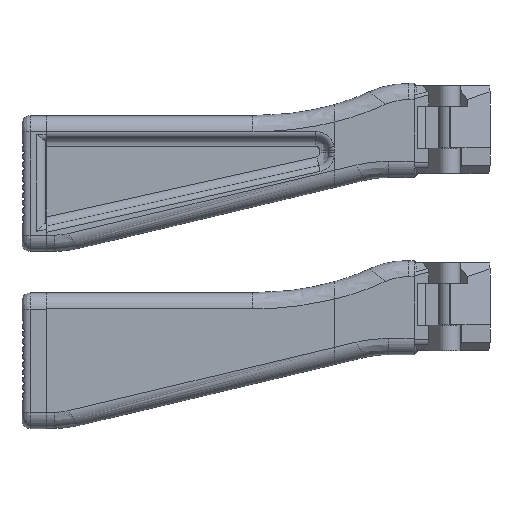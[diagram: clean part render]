
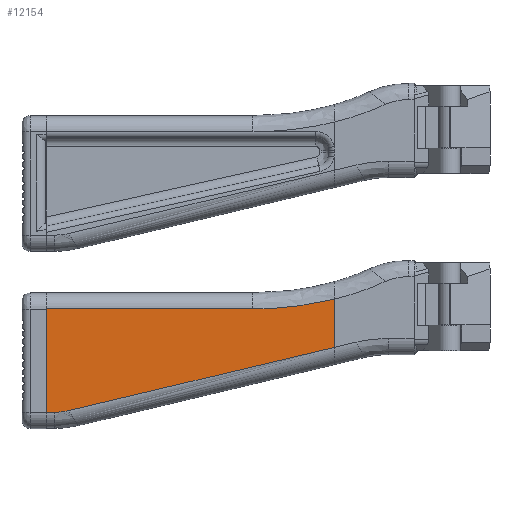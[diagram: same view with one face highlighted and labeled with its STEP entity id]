
A CAD part, top view. The second image highlights one B-rep face of the part: STEP entity #12154.
In plain terms, the highlighted planar face has unit normal (0, 0, 1).
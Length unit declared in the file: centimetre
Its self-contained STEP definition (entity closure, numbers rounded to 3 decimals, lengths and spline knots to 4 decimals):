
#967=ELLIPSE($,#13110,2.4171,1.5);
#968=ELLIPSE($,#13111,13.6966,8.5);
#1830=FACE_OUTER_BOUND($,#2569,.T.);
#2569=EDGE_LOOP($,(#9771,#9772,#9773,#9774,#9775,#9776,#9777));
#3414=LINE($,#23897,#4329);
#3415=LINE($,#23899,#4330);
#3416=LINE($,#23903,#4331);
#3417=LINE($,#23905,#4332);
#3418=LINE($,#23908,#4333);
#4329=VECTOR($,#15317,6.4209);
#4330=VECTOR($,#15318,0.5316);
#4331=VECTOR($,#15321,16.9639);
#4332=VECTOR($,#15322,2.992);
#4333=VECTOR($,#15325,12.8428);
#5404=VERTEX_POINT($,#23895);
#5405=VERTEX_POINT($,#23896);
#5406=VERTEX_POINT($,#23898);
#5407=VERTEX_POINT($,#23900);
#5408=VERTEX_POINT($,#23902);
#5409=VERTEX_POINT($,#23904);
#5410=VERTEX_POINT($,#23906);
#6950=EDGE_CURVE($,#5404,#5405,#3414,.F.);
#6951=EDGE_CURVE($,#5404,#5406,#3415,.T.);
#6952=EDGE_CURVE($,#5406,#5407,#967,.T.);
#6953=EDGE_CURVE($,#5407,#5408,#3416,.T.);
#6954=EDGE_CURVE($,#5408,#5409,#3417,.T.);
#6955=EDGE_CURVE($,#5409,#5410,#968,.T.);
#6956=EDGE_CURVE($,#5410,#5405,#3418,.T.);
#9771=ORIENTED_EDGE($,*,*,#6950,.F.);
#9772=ORIENTED_EDGE($,*,*,#6951,.T.);
#9773=ORIENTED_EDGE($,*,*,#6952,.T.);
#9774=ORIENTED_EDGE($,*,*,#6953,.T.);
#9775=ORIENTED_EDGE($,*,*,#6954,.T.);
#9776=ORIENTED_EDGE($,*,*,#6955,.T.);
#9777=ORIENTED_EDGE($,*,*,#6956,.T.);
#11653=PLANE($,#13109);
#12154=ADVANCED_FACE($,(#1830),#11653,.T.);
#13109=AXIS2_PLACEMENT_3D($,#23894,#15315,#15316);
#13110=AXIS2_PLACEMENT_3D($,#23901,#15319,#15320);
#13111=AXIS2_PLACEMENT_3D($,#23907,#15323,#15324);
#15315=DIRECTION('center_axis',(0.,0.,
1.));
#15316=DIRECTION('ref_axis',(1.,0.,0.));
#15317=DIRECTION($,(0.,-1.,0.));
#15318=DIRECTION($,(1.,0.,0.));
#15319=DIRECTION('center_axis',(0.,0.,
1.));
#15320=DIRECTION('ref_axis',(1.,0.,0.));
#15321=DIRECTION($,(0.973,0.232,0.));
#15322=DIRECTION($,(0.,1.,0.));
#15323=DIRECTION('center_axis',(0.,0.,
-1.));
#15324=DIRECTION('ref_axis',(-1.,0.,0.));
#15325=DIRECTION($,(-1.,0.,0.));
#23894=CARTESIAN_POINT('Origin',(-24.6928,-5.5542,21.6357));
#23895=CARTESIAN_POINT('',(-47.3633,-14.9752,21.6357));
#23896=CARTESIAN_POINT('',(-47.3633,-8.5542,21.6357));
#23897=CARTESIAN_POINT($,(-47.3633,-10.0146,21.6357));
#23898=CARTESIAN_POINT('',(-46.8317,-14.9752,21.6357));
#23899=CARTESIAN_POINT($,(-28.0525,-14.9752,21.6357));
#23900=CARTESIAN_POINT('',(-45.9657,-14.8756,21.6357));
#23901=CARTESIAN_POINT('Origin',(-46.8317,-13.4752,21.6357));
#23902=CARTESIAN_POINT('',(-29.4633,-10.9456,21.6357));
#23903=CARTESIAN_POINT($,(-26.3884,-10.2134,21.6357));
#23904=CARTESIAN_POINT('',(-29.4633,-7.9536,21.6357));
#23905=CARTESIAN_POINT($,(-29.4633,-8.677,21.6357));
#23906=CARTESIAN_POINT('',(-34.5205,-8.5542,21.6357));
#23907=CARTESIAN_POINT('Origin',(-34.5205,-0.0542,21.6357));
#23908=CARTESIAN_POINT($,(-24.6928,-8.5542,21.6357));
